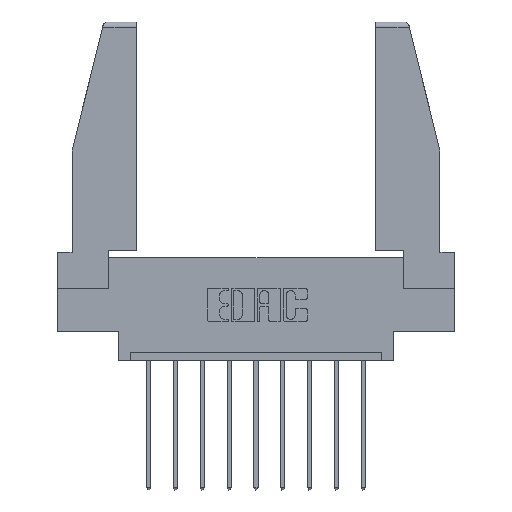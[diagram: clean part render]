
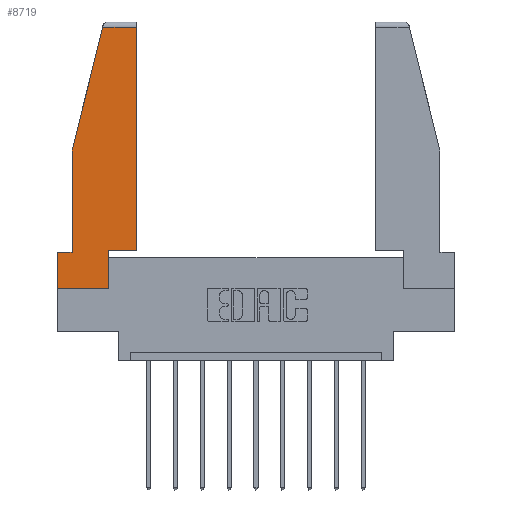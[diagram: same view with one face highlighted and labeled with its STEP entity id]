
A CAD part, top view. The second image highlights one B-rep face of the part: STEP entity #8719.
In plain terms, the highlighted planar face has unit normal (0, 0, 1).
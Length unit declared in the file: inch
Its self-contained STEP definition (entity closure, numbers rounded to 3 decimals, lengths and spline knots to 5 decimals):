
#94 = DIRECTION ( 'NONE',  ( 0., -1., 0. ) ) ;
#548 = CARTESIAN_POINT ( 'NONE',  ( 0., 0.21, 0. ) ) ;
#592 = DIRECTION ( 'NONE',  ( 0., -1., 0. ) ) ;
#876 = LINE ( 'NONE', #548, #10038 ) ;
#901 = CARTESIAN_POINT ( 'NONE',  ( 0.297, 0., 0. ) ) ;
#968 = ORIENTED_EDGE ( 'NONE', *, *, #1650, .T. ) ;
#1070 = DIRECTION ( 'NONE',  ( 0., 1., 0. ) ) ;
#1225 = CARTESIAN_POINT ( 'NONE',  ( 0., 0., 0. ) ) ;
#1377 = LINE ( 'NONE', #11615, #3807 ) ;
#1650 = EDGE_CURVE ( 'NONE', #8561, #11874, #11927, .T. ) ;
#2438 = CARTESIAN_POINT ( 'NONE',  ( 0.086, 0.21, 0. ) ) ;
#2552 = LINE ( 'NONE', #5527, #10234 ) ;
#3001 = CARTESIAN_POINT ( 'NONE',  ( 0.086, 0.8, 0. ) ) ;
#3068 = LINE ( 'NONE', #9214, #5496 ) ;
#3223 = CARTESIAN_POINT ( 'NONE',  ( 0.297, 0., 0. ) ) ;
#3276 = VECTOR ( 'NONE', #13471, 39.37008 ) ;
#3338 = ORIENTED_EDGE ( 'NONE', *, *, #3711, .T. ) ;
#3642 = VERTEX_POINT ( 'NONE', #3001 ) ;
#3711 = EDGE_CURVE ( 'NONE', #5277, #5492, #6596, .T. ) ;
#3782 = LINE ( 'NONE', #6595, #12113 ) ;
#3807 = VECTOR ( 'NONE', #94, 39.37008 ) ;
#3871 = ORIENTED_EDGE ( 'NONE', *, *, #4500, .T. ) ;
#4082 = DIRECTION ( 'NONE',  ( 0., 0., 1. ) ) ;
#4140 = CARTESIAN_POINT ( 'NONE',  ( 0., 0., 0. ) ) ;
#4353 = VERTEX_POINT ( 'NONE', #7378 ) ;
#4360 = DIRECTION ( 'NONE',  ( -0.239, -0.971, 0. ) ) ;
#4500 = EDGE_CURVE ( 'NONE', #7286, #4986, #2552, .T. ) ;
#4916 = DIRECTION ( 'NONE',  ( -1., 0., 0. ) ) ;
#4986 = VERTEX_POINT ( 'NONE', #6712 ) ;
#5277 = VERTEX_POINT ( 'NONE', #2438 ) ;
#5367 = ORIENTED_EDGE ( 'NONE', *, *, #12568, .T. ) ;
#5492 = VERTEX_POINT ( 'NONE', #9746 ) ;
#5496 = VECTOR ( 'NONE', #4916, 39.37008 ) ;
#5527 = CARTESIAN_POINT ( 'NONE',  ( 0.461, 0.223, 0. ) ) ;
#5656 = LINE ( 'NONE', #13475, #6424 ) ;
#5988 = CARTESIAN_POINT ( 'NONE',  ( 0., 0., 0. ) ) ;
#6424 = VECTOR ( 'NONE', #4360, 39.37008 ) ;
#6595 = CARTESIAN_POINT ( 'NONE',  ( 0.297, 0.223, 0. ) ) ;
#6596 = LINE ( 'NONE', #7275, #12175 ) ;
#6700 = CARTESIAN_POINT ( 'NONE',  ( 0.461, 0.223, 0. ) ) ;
#6712 = CARTESIAN_POINT ( 'NONE',  ( 0.461, 1.52, 0. ) ) ;
#6912 = ORIENTED_EDGE ( 'NONE', *, *, #8586, .T. ) ;
#7143 = ORIENTED_EDGE ( 'NONE', *, *, #8427, .T. ) ;
#7275 = CARTESIAN_POINT ( 'NONE',  ( 0., 0.21, 0. ) ) ;
#7286 = VERTEX_POINT ( 'NONE', #6700 ) ;
#7378 = CARTESIAN_POINT ( 'NONE',  ( 0.297, 0.223, 0. ) ) ;
#7602 = DIRECTION ( 'NONE',  ( 0., 1., 0. ) ) ;
#8427 = EDGE_CURVE ( 'NONE', #4986, #10592, #3068, .T. ) ;
#8495 = ORIENTED_EDGE ( 'NONE', *, *, #11948, .T. ) ;
#8508 = DIRECTION ( 'NONE',  ( -1., 0., 0. ) ) ;
#8561 = VERTEX_POINT ( 'NONE', #1225 ) ;
#8584 = ORIENTED_EDGE ( 'NONE', *, *, #12160, .T. ) ;
#8586 = EDGE_CURVE ( 'NONE', #10592, #3642, #5656, .T. ) ;
#8719 = ADVANCED_FACE ( 'NONE', ( #9922 ), #13459, .T. ) ;
#8850 = VECTOR ( 'NONE', #1070, 39.37008 ) ;
#9214 = CARTESIAN_POINT ( 'NONE',  ( 0., 1.52, 0. ) ) ;
#9746 = CARTESIAN_POINT ( 'NONE',  ( 0., 0.21, 0. ) ) ;
#9769 = DIRECTION ( 'NONE',  ( 1., 0., 0. ) ) ;
#9922 = FACE_OUTER_BOUND ( 'NONE', #10290, .T. ) ;
#10038 = VECTOR ( 'NONE', #592, 39.37008 ) ;
#10234 = VECTOR ( 'NONE', #7602, 39.37008 ) ;
#10290 = EDGE_LOOP ( 'NONE', ( #3871, #7143, #6912, #8495, #3338, #8584, #968, #11764, #5367 ) ) ;
#10592 = VERTEX_POINT ( 'NONE', #11250 ) ;
#11250 = CARTESIAN_POINT ( 'NONE',  ( 0.2636, 1.52, 0. ) ) ;
#11385 = DIRECTION ( 'NONE',  ( 1., 0., 0. ) ) ;
#11600 = LINE ( 'NONE', #3223, #8850 ) ;
#11615 = CARTESIAN_POINT ( 'NONE',  ( 0.086, 0.8, 0. ) ) ;
#11764 = ORIENTED_EDGE ( 'NONE', *, *, #13474, .T. ) ;
#11874 = VERTEX_POINT ( 'NONE', #901 ) ;
#11927 = LINE ( 'NONE', #4140, #3276 ) ;
#11948 = EDGE_CURVE ( 'NONE', #3642, #5277, #1377, .T. ) ;
#12113 = VECTOR ( 'NONE', #9769, 39.37008 ) ;
#12160 = EDGE_CURVE ( 'NONE', #5492, #8561, #876, .T. ) ;
#12175 = VECTOR ( 'NONE', #8508, 39.37008 ) ;
#12300 = AXIS2_PLACEMENT_3D ( 'NONE', #5988, #4082, #11385 ) ;
#12568 = EDGE_CURVE ( 'NONE', #4353, #7286, #3782, .T. ) ;
#13459 = PLANE ( 'NONE',  #12300 ) ;
#13471 = DIRECTION ( 'NONE',  ( 1., 0., 0. ) ) ;
#13474 = EDGE_CURVE ( 'NONE', #11874, #4353, #11600, .T. ) ;
#13475 = CARTESIAN_POINT ( 'NONE',  ( 0.271, 1.55, 0. ) ) ;
